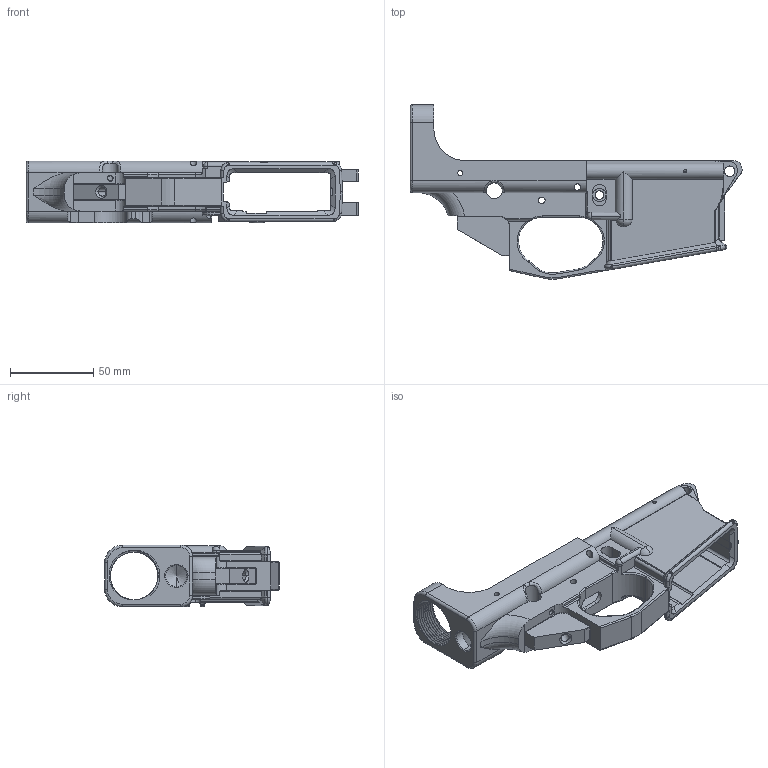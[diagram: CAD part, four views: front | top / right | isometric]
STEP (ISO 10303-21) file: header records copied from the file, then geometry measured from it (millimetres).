
FILE_DESCRIPTION(('FreeCAD Model'),'2;1');
FILE_NAME('AR-15-Lower-V5.step', '2016-04-03T13:25:37',('Author'),(''), 'Open CASCADE STEP processor 6.8','FreeCAD','Unknown');
FILE_SCHEMA(('AUTOMOTIVE_DESIGN_CC2 { 1 2 10303 214 -1 1 5 4 }'));
Products named in the file (1): Pocket003
Bounding box: 199.55 x 104.92 x 37.19 mm (x, y, z)
Volume: 136664.2 mm3; surface area: 59068.1 mm2
Topology: 1 solids, 1 shells, 919 faces, 2535 edges, 1632 vertices
Faces by surface type: plane 443, cylinder 250, bspline 154, torus 51, cone 12, sphere 7, revolution 2
Entity records: 119441 total; most frequent: CARTESIAN_POINT 75253, DIRECTION 6179, ORIENTED_EDGE 5048, PCURVE 5046, DEFINITIONAL_REPRESENTATION 5046, LINE 3633, VECTOR 3633, B_SPLINE_CURVE_WITH_KNOTS 3180
